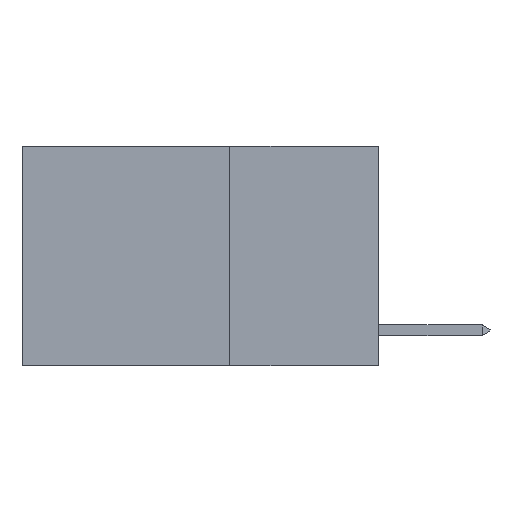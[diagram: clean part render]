
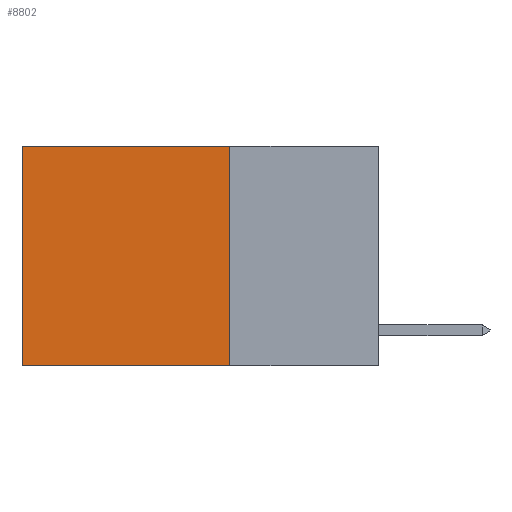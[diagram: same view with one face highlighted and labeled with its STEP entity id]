
A CAD part, left-side view. The second image highlights one B-rep face of the part: STEP entity #8802.
In plain terms, the highlighted planar face has unit normal (-1, 0, 0).
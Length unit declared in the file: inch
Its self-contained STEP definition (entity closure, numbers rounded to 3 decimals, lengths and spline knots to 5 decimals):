
#1594 = CARTESIAN_POINT ( 'NONE',  ( 0.2625, 0.6, -0.37 ) ) ;
#1597 = AXIS2_PLACEMENT_3D ( 'NONE', #5967, #9205, #7041 ) ;
#1982 = ORIENTED_EDGE ( 'NONE', *, *, #3705, .F. ) ;
#2288 = VECTOR ( 'NONE', #10717, 39.37008 ) ;
#2455 = EDGE_CURVE ( 'NONE', #11411, #4159, #14017, .T. ) ;
#2953 = LINE ( 'NONE', #10314, #13776 ) ;
#3546 = ORIENTED_EDGE ( 'NONE', *, *, #9892, .T. ) ;
#3705 = EDGE_CURVE ( 'NONE', #12326, #4159, #7997, .T. ) ;
#3869 = VECTOR ( 'NONE', #12799, 39.37008 ) ;
#4116 = CARTESIAN_POINT ( 'NONE',  ( 0.2625, 0.25, 0. ) ) ;
#4159 = VERTEX_POINT ( 'NONE', #1594 ) ;
#5061 = EDGE_LOOP ( 'NONE', ( #11582, #1982, #8436, #3546 ) ) ;
#5967 = CARTESIAN_POINT ( 'NONE',  ( 0.2625, 0.25, 0. ) ) ;
#6989 = LINE ( 'NONE', #4116, #2288 ) ;
#7041 = DIRECTION ( 'NONE',  ( 0., 0., -1. ) ) ;
#7082 = DIRECTION ( 'NONE',  ( 0., 1., 0. ) ) ;
#7997 = LINE ( 'NONE', #13573, #8481 ) ;
#8116 = VERTEX_POINT ( 'NONE', #12483 ) ;
#8436 = ORIENTED_EDGE ( 'NONE', *, *, #9308, .F. ) ;
#8481 = VECTOR ( 'NONE', #7082, 39.37008 ) ;
#8802 = ADVANCED_FACE ( 'NONE', ( #11817 ), #10171, .F. ) ;
#9205 = DIRECTION ( 'NONE',  ( 1., 0., 0. ) ) ;
#9308 = EDGE_CURVE ( 'NONE', #8116, #12326, #6989, .T. ) ;
#9892 = EDGE_CURVE ( 'NONE', #8116, #11411, #2953, .T. ) ;
#10171 = PLANE ( 'NONE',  #1597 ) ;
#10314 = CARTESIAN_POINT ( 'NONE',  ( 0.2625, 0.25, 0. ) ) ;
#10717 = DIRECTION ( 'NONE',  ( 0., 0., -1. ) ) ;
#11089 = CARTESIAN_POINT ( 'NONE',  ( 0.2625, 0.6, 0. ) ) ;
#11411 = VERTEX_POINT ( 'NONE', #11089 ) ;
#11582 = ORIENTED_EDGE ( 'NONE', *, *, #2455, .T. ) ;
#11729 = CARTESIAN_POINT ( 'NONE',  ( 0.2625, 0.6, 0. ) ) ;
#11817 = FACE_OUTER_BOUND ( 'NONE', #5061, .T. ) ;
#12326 = VERTEX_POINT ( 'NONE', #13920 ) ;
#12412 = DIRECTION ( 'NONE',  ( 0., 1., 0. ) ) ;
#12483 = CARTESIAN_POINT ( 'NONE',  ( 0.2625, 0.25, 0. ) ) ;
#12799 = DIRECTION ( 'NONE',  ( 0., 0., -1. ) ) ;
#13573 = CARTESIAN_POINT ( 'NONE',  ( 0.2625, 0.25, -0.37 ) ) ;
#13776 = VECTOR ( 'NONE', #12412, 39.37008 ) ;
#13920 = CARTESIAN_POINT ( 'NONE',  ( 0.2625, 0.25, -0.37 ) ) ;
#14017 = LINE ( 'NONE', #11729, #3869 ) ;
